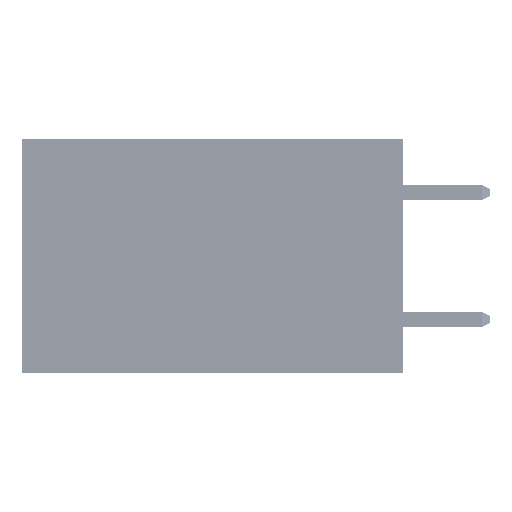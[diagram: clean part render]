
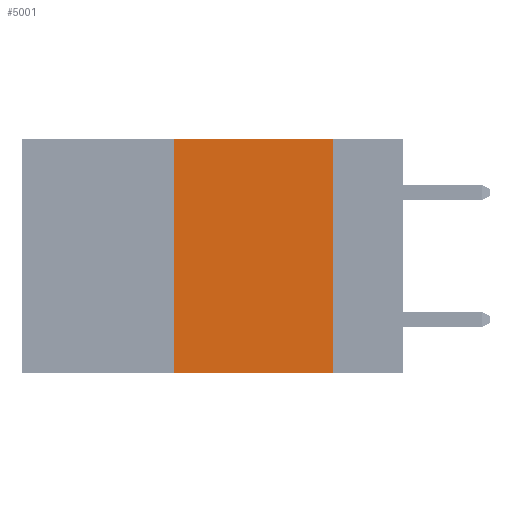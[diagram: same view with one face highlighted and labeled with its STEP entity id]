
A CAD part, left-side view. The second image highlights one B-rep face of the part: STEP entity #5001.
In plain terms, the highlighted planar face has unit normal (-1, 0, 0).
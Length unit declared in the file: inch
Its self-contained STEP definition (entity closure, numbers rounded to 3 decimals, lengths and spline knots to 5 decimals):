
#575 = VECTOR ( 'NONE', #36866, 39.37008 ) ;
#784 = EDGE_LOOP ( 'NONE', ( #41840, #9147, #22797, #24504 ) ) ;
#4240 = CARTESIAN_POINT ( 'NONE',  ( 0., 0.6, 0. ) ) ;
#4470 = CARTESIAN_POINT ( 'NONE',  ( 0., 0.11, 0. ) ) ;
#5001 = ADVANCED_FACE ( 'NONE', ( #7071 ), #10328, .F. ) ;
#5263 = VECTOR ( 'NONE', #8640, 39.37008 ) ;
#5916 = CARTESIAN_POINT ( 'NONE',  ( 0., 0.11, 0. ) ) ;
#6140 = CARTESIAN_POINT ( 'NONE',  ( 0., 0.36, 0. ) ) ;
#6730 = VECTOR ( 'NONE', #16553, 39.37008 ) ;
#7071 = FACE_OUTER_BOUND ( 'NONE', #784, .T. ) ;
#7793 = CARTESIAN_POINT ( 'NONE',  ( 0., 0.36, -0.37 ) ) ;
#8640 = DIRECTION ( 'NONE',  ( 0., 0., -1. ) ) ;
#9147 = ORIENTED_EDGE ( 'NONE', *, *, #20865, .F. ) ;
#10328 = PLANE ( 'NONE',  #48112 ) ;
#11133 = LINE ( 'NONE', #39650, #28817 ) ;
#11359 = DIRECTION ( 'NONE',  ( 0., 0., -1. ) ) ;
#11774 = LINE ( 'NONE', #4470, #5263 ) ;
#13887 = DIRECTION ( 'NONE',  ( 0., -1., 0. ) ) ;
#16553 = DIRECTION ( 'NONE',  ( 0., -1., 0. ) ) ;
#20865 = EDGE_CURVE ( 'NONE', #43794, #26717, #11133, .T. ) ;
#22054 = LINE ( 'NONE', #31705, #6730 ) ;
#22797 = ORIENTED_EDGE ( 'NONE', *, *, #33542, .F. ) ;
#23899 = EDGE_CURVE ( 'NONE', #46252, #42301, #22054, .T. ) ;
#24504 = ORIENTED_EDGE ( 'NONE', *, *, #23899, .T. ) ;
#26570 = CARTESIAN_POINT ( 'NONE',  ( 0., 0.11, -0.37 ) ) ;
#26717 = VERTEX_POINT ( 'NONE', #5916 ) ;
#26844 = DIRECTION ( 'NONE',  ( 1., 0., 0. ) ) ;
#28817 = VECTOR ( 'NONE', #13887, 39.37008 ) ;
#31705 = CARTESIAN_POINT ( 'NONE',  ( 0., 0.6, -0.37 ) ) ;
#33542 = EDGE_CURVE ( 'NONE', #46252, #43794, #45944, .T. ) ;
#33851 = EDGE_CURVE ( 'NONE', #26717, #42301, #11774, .T. ) ;
#36866 = DIRECTION ( 'NONE',  ( 0., 0., 1. ) ) ;
#39650 = CARTESIAN_POINT ( 'NONE',  ( 0., 0.6, 0. ) ) ;
#41840 = ORIENTED_EDGE ( 'NONE', *, *, #33851, .F. ) ;
#42301 = VERTEX_POINT ( 'NONE', #26570 ) ;
#43794 = VERTEX_POINT ( 'NONE', #6140 ) ;
#45944 = LINE ( 'NONE', #47969, #575 ) ;
#46252 = VERTEX_POINT ( 'NONE', #7793 ) ;
#47969 = CARTESIAN_POINT ( 'NONE',  ( 0., 0.36, 0. ) ) ;
#48112 = AXIS2_PLACEMENT_3D ( 'NONE', #4240, #26844, #11359 ) ;
